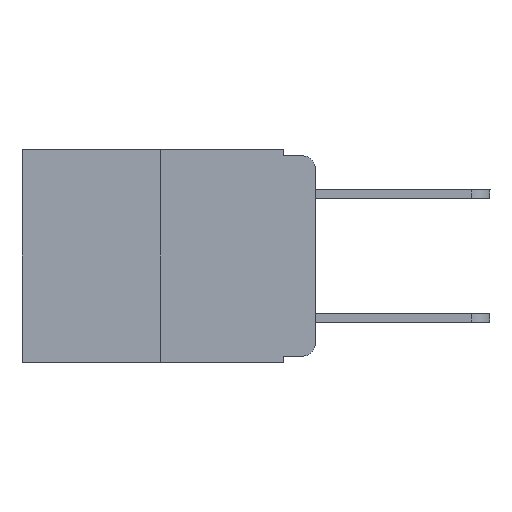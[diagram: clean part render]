
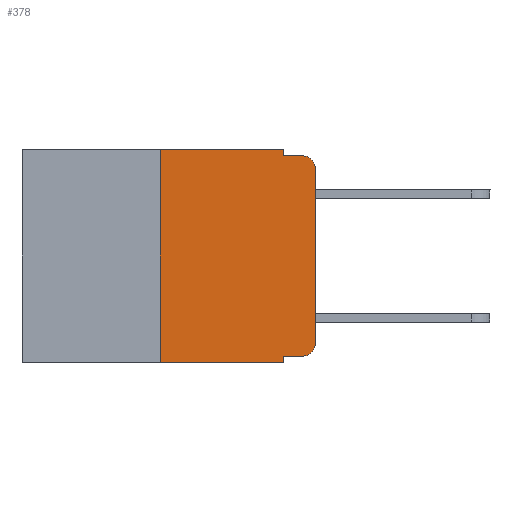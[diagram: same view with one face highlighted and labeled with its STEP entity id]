
A CAD part, left-side view. The second image highlights one B-rep face of the part: STEP entity #378.
In plain terms, the highlighted planar face has unit normal (-1, 0, 0).
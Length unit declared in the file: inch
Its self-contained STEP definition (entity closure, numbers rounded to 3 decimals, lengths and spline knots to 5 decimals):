
#341 = DIRECTION ( 'NONE',  ( 1., 0., 0. ) ) ;
#378 = ADVANCED_FACE ( 'NONE', ( #454 ), #12792, .F. ) ;
#419 = EDGE_CURVE ( 'NONE', #12050, #23933, #19166, .T. ) ;
#454 = FACE_OUTER_BOUND ( 'NONE', #2959, .T. ) ;
#1000 = ORIENTED_EDGE ( 'NONE', *, *, #8712, .T. ) ;
#1426 = DIRECTION ( 'NONE',  ( 0., -1., 0. ) ) ;
#2326 = VECTOR ( 'NONE', #4739, 39.37008 ) ;
#2647 = VECTOR ( 'NONE', #1426, 39.37008 ) ;
#2665 = ORIENTED_EDGE ( 'NONE', *, *, #5258, .F. ) ;
#2887 = LINE ( 'NONE', #9044, #2647 ) ;
#2932 = DIRECTION ( 'NONE',  ( 0., 0., 1. ) ) ;
#2959 = EDGE_LOOP ( 'NONE', ( #7145, #24525, #2665, #24391, #18306, #21329, #1000, #25026, #8088, #17221 ) ) ;
#3569 = AXIS2_PLACEMENT_3D ( 'NONE', #5060, #9556, #15551 ) ;
#4158 = CARTESIAN_POINT ( 'NONE',  ( 0., 0.25, 0. ) ) ;
#4174 = LINE ( 'NONE', #4429, #16143 ) ;
#4307 = VECTOR ( 'NONE', #9531, 39.37008 ) ;
#4429 = CARTESIAN_POINT ( 'NONE',  ( 0., 0.473, -0.343 ) ) ;
#4656 = EDGE_CURVE ( 'NONE', #16685, #7453, #5963, .T. ) ;
#4739 = DIRECTION ( 'NONE',  ( 0., 0., -1. ) ) ;
#5027 = VERTEX_POINT ( 'NONE', #20301 ) ;
#5060 = CARTESIAN_POINT ( 'NONE',  ( 0., 0.02, -0.03 ) ) ;
#5258 = EDGE_CURVE ( 'NONE', #11326, #17993, #2887, .T. ) ;
#5320 = CARTESIAN_POINT ( 'NONE',  ( 0., 0.051, -0.01 ) ) ;
#5826 = CARTESIAN_POINT ( 'NONE',  ( 0., 0.02, -0.313 ) ) ;
#5963 = LINE ( 'NONE', #24025, #10551 ) ;
#6587 = LINE ( 'NONE', #20460, #2326 ) ;
#6671 = CARTESIAN_POINT ( 'NONE',  ( 0., 0.25, 0. ) ) ;
#6730 = DIRECTION ( 'NONE',  ( 0., -1., 0. ) ) ;
#7145 = ORIENTED_EDGE ( 'NONE', *, *, #419, .T. ) ;
#7453 = VERTEX_POINT ( 'NONE', #15960 ) ;
#7528 = LINE ( 'NONE', #23235, #4307 ) ;
#8088 = ORIENTED_EDGE ( 'NONE', *, *, #4656, .T. ) ;
#8320 = DIRECTION ( 'NONE',  ( 0., 0., -1. ) ) ;
#8712 = EDGE_CURVE ( 'NONE', #19034, #5027, #4174, .T. ) ;
#9044 = CARTESIAN_POINT ( 'NONE',  ( 0., 0.051, -0.01 ) ) ;
#9531 = DIRECTION ( 'NONE',  ( 0., 0., -1. ) ) ;
#9556 = DIRECTION ( 'NONE',  ( -1., 0., 0. ) ) ;
#9780 = AXIS2_PLACEMENT_3D ( 'NONE', #22295, #341, #8320 ) ;
#10551 = VECTOR ( 'NONE', #12427, 39.37008 ) ;
#10569 = CARTESIAN_POINT ( 'NONE',  ( 0., 0.051, -0.333 ) ) ;
#10823 = CARTESIAN_POINT ( 'NONE',  ( 0., 0., -0.03 ) ) ;
#11241 = VERTEX_POINT ( 'NONE', #4158 ) ;
#11326 = VERTEX_POINT ( 'NONE', #5320 ) ;
#11547 = CIRCLE ( 'NONE', #3569, 0.02 ) ;
#11549 = EDGE_CURVE ( 'NONE', #7453, #12050, #17246, .T. ) ;
#12050 = VERTEX_POINT ( 'NONE', #19274 ) ;
#12427 = DIRECTION ( 'NONE',  ( 0., -1., 0. ) ) ;
#12792 = PLANE ( 'NONE',  #9780 ) ;
#12917 = CARTESIAN_POINT ( 'NONE',  ( 0., 0., 0. ) ) ;
#13579 = DIRECTION ( 'NONE',  ( -1., 0., 0. ) ) ;
#15347 = CARTESIAN_POINT ( 'NONE',  ( 0., 0.25, -0.343 ) ) ;
#15384 = EDGE_CURVE ( 'NONE', #11241, #20425, #16330, .T. ) ;
#15551 = DIRECTION ( 'NONE',  ( 0., 0., -1. ) ) ;
#15679 = VECTOR ( 'NONE', #6730, 39.37008 ) ;
#15960 = CARTESIAN_POINT ( 'NONE',  ( 0., 0.02, -0.333 ) ) ;
#16143 = VECTOR ( 'NONE', #16242, 39.37008 ) ;
#16242 = DIRECTION ( 'NONE',  ( 0., -1., 0. ) ) ;
#16330 = LINE ( 'NONE', #24652, #15679 ) ;
#16371 = EDGE_CURVE ( 'NONE', #23933, #17993, #11547, .T. ) ;
#16685 = VERTEX_POINT ( 'NONE', #10569 ) ;
#17221 = ORIENTED_EDGE ( 'NONE', *, *, #11549, .T. ) ;
#17246 = CIRCLE ( 'NONE', #24718, 0.02 ) ;
#17585 = EDGE_CURVE ( 'NONE', #19034, #11241, #18725, .T. ) ;
#17993 = VERTEX_POINT ( 'NONE', #20606 ) ;
#18306 = ORIENTED_EDGE ( 'NONE', *, *, #15384, .F. ) ;
#18725 = LINE ( 'NONE', #6671, #24804 ) ;
#19034 = VERTEX_POINT ( 'NONE', #15347 ) ;
#19166 = LINE ( 'NONE', #12917, #23109 ) ;
#19274 = CARTESIAN_POINT ( 'NONE',  ( 0., 0., -0.313 ) ) ;
#20165 = DIRECTION ( 'NONE',  ( 0., 0., 1. ) ) ;
#20301 = CARTESIAN_POINT ( 'NONE',  ( 0., 0.051, -0.343 ) ) ;
#20344 = EDGE_CURVE ( 'NONE', #20425, #11326, #6587, .T. ) ;
#20425 = VERTEX_POINT ( 'NONE', #22796 ) ;
#20460 = CARTESIAN_POINT ( 'NONE',  ( 0., 0.051, 0. ) ) ;
#20606 = CARTESIAN_POINT ( 'NONE',  ( 0., 0.02, -0.01 ) ) ;
#21329 = ORIENTED_EDGE ( 'NONE', *, *, #17585, .F. ) ;
#22295 = CARTESIAN_POINT ( 'NONE',  ( 0., 0.473, 0. ) ) ;
#22629 = EDGE_CURVE ( 'NONE', #16685, #5027, #7528, .T. ) ;
#22796 = CARTESIAN_POINT ( 'NONE',  ( 0., 0.051, 0. ) ) ;
#23109 = VECTOR ( 'NONE', #2932, 39.37008 ) ;
#23235 = CARTESIAN_POINT ( 'NONE',  ( 0., 0.051, 0. ) ) ;
#23863 = DIRECTION ( 'NONE',  ( 0., 0., -1. ) ) ;
#23933 = VERTEX_POINT ( 'NONE', #10823 ) ;
#24025 = CARTESIAN_POINT ( 'NONE',  ( 0., 0.051, -0.333 ) ) ;
#24391 = ORIENTED_EDGE ( 'NONE', *, *, #20344, .F. ) ;
#24525 = ORIENTED_EDGE ( 'NONE', *, *, #16371, .T. ) ;
#24652 = CARTESIAN_POINT ( 'NONE',  ( 0., 0.473, 0. ) ) ;
#24718 = AXIS2_PLACEMENT_3D ( 'NONE', #5826, #13579, #23863 ) ;
#24804 = VECTOR ( 'NONE', #20165, 39.37008 ) ;
#25026 = ORIENTED_EDGE ( 'NONE', *, *, #22629, .F. ) ;
